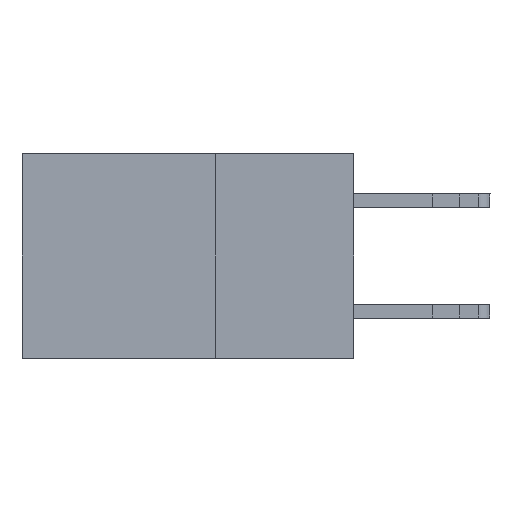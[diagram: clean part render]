
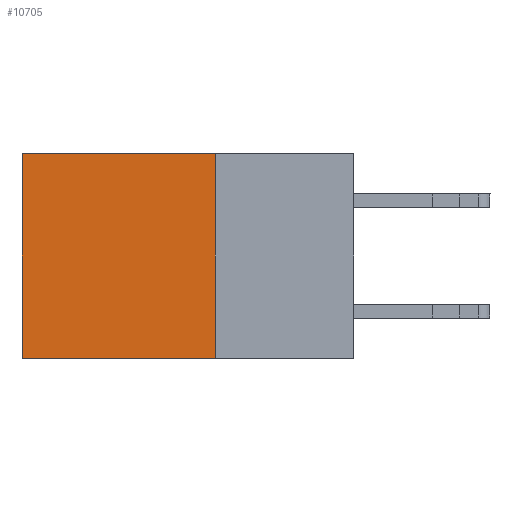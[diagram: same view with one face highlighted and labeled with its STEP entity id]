
A CAD part, left-side view. The second image highlights one B-rep face of the part: STEP entity #10705.
In plain terms, the highlighted planar face has unit normal (-1, 0, 0).
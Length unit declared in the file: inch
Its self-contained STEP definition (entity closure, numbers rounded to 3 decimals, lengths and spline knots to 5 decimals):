
#375 = VERTEX_POINT ( 'NONE', #699 ) ;
#452 = ORIENTED_EDGE ( 'NONE', *, *, #15321, .F. ) ;
#699 = CARTESIAN_POINT ( 'NONE',  ( 0.2875, 0.6, 0. ) ) ;
#935 = VECTOR ( 'NONE', #6902, 39.37008 ) ;
#2577 = LINE ( 'NONE', #8825, #5520 ) ;
#3553 = VECTOR ( 'NONE', #8208, 39.37008 ) ;
#4381 = CARTESIAN_POINT ( 'NONE',  ( 0.2875, 0.25, 0. ) ) ;
#4700 = ORIENTED_EDGE ( 'NONE', *, *, #15004, .T. ) ;
#5520 = VECTOR ( 'NONE', #7280, 39.37008 ) ;
#6420 = VECTOR ( 'NONE', #17301, 39.37008 ) ;
#6562 = CARTESIAN_POINT ( 'NONE',  ( 0.2875, 0.25, 0. ) ) ;
#6902 = DIRECTION ( 'NONE',  ( 0., 0., -1. ) ) ;
#7280 = DIRECTION ( 'NONE',  ( 0., 1., 0. ) ) ;
#7978 = ORIENTED_EDGE ( 'NONE', *, *, #14702, .T. ) ;
#8207 = EDGE_CURVE ( 'NONE', #16388, #15217, #18950, .T. ) ;
#8208 = DIRECTION ( 'NONE',  ( 0., 1., 0. ) ) ;
#8825 = CARTESIAN_POINT ( 'NONE',  ( 0.2875, 0.25, -0.37 ) ) ;
#9573 = CARTESIAN_POINT ( 'NONE',  ( 0.2875, 0.25, 0. ) ) ;
#10458 = DIRECTION ( 'NONE',  ( 1., 0., 0. ) ) ;
#10705 = ADVANCED_FACE ( 'NONE', ( #18293 ), #15211, .F. ) ;
#11754 = LINE ( 'NONE', #17940, #935 ) ;
#13581 = CARTESIAN_POINT ( 'NONE',  ( 0.2875, 0.25, -0.37 ) ) ;
#14702 = EDGE_CURVE ( 'NONE', #375, #15242, #11754, .T. ) ;
#15004 = EDGE_CURVE ( 'NONE', #16388, #375, #17703, .T. ) ;
#15211 = PLANE ( 'NONE',  #15531 ) ;
#15217 = VERTEX_POINT ( 'NONE', #13581 ) ;
#15242 = VERTEX_POINT ( 'NONE', #16773 ) ;
#15321 = EDGE_CURVE ( 'NONE', #15217, #15242, #2577, .T. ) ;
#15531 = AXIS2_PLACEMENT_3D ( 'NONE', #4381, #10458, #16743 ) ;
#16388 = VERTEX_POINT ( 'NONE', #9573 ) ;
#16743 = DIRECTION ( 'NONE',  ( 0., 0., -1. ) ) ;
#16773 = CARTESIAN_POINT ( 'NONE',  ( 0.2875, 0.6, -0.37 ) ) ;
#16798 = ORIENTED_EDGE ( 'NONE', *, *, #8207, .F. ) ;
#17190 = EDGE_LOOP ( 'NONE', ( #7978, #452, #16798, #4700 ) ) ;
#17301 = DIRECTION ( 'NONE',  ( 0., 0., -1. ) ) ;
#17703 = LINE ( 'NONE', #6562, #3553 ) ;
#17940 = CARTESIAN_POINT ( 'NONE',  ( 0.2875, 0.6, 0. ) ) ;
#18293 = FACE_OUTER_BOUND ( 'NONE', #17190, .T. ) ;
#18740 = CARTESIAN_POINT ( 'NONE',  ( 0.2875, 0.25, 0. ) ) ;
#18950 = LINE ( 'NONE', #18740, #6420 ) ;
